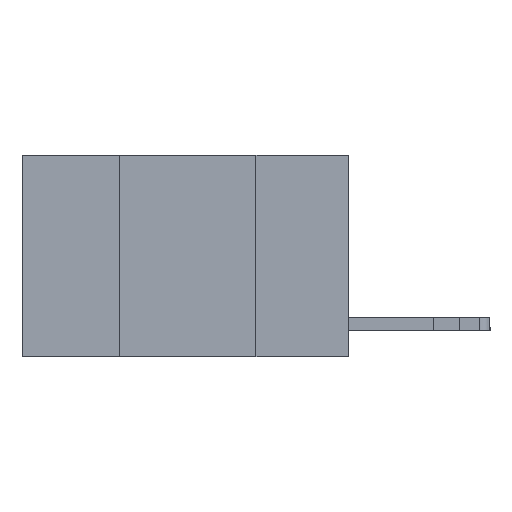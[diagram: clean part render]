
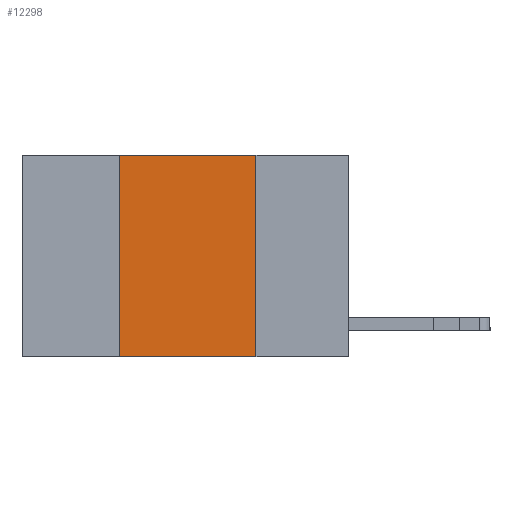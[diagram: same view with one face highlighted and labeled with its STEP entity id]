
A CAD part, left-side view. The second image highlights one B-rep face of the part: STEP entity #12298.
In plain terms, the highlighted planar face has unit normal (-1, 0, 0).
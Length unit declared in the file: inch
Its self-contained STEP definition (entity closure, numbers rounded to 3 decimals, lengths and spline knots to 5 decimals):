
#1018 = ORIENTED_EDGE ( 'NONE', *, *, #19228, .F. ) ;
#1240 = CARTESIAN_POINT ( 'NONE',  ( 0., 0.17, -0.37 ) ) ;
#2890 = VECTOR ( 'NONE', #11458, 39.37008 ) ;
#2961 = ORIENTED_EDGE ( 'NONE', *, *, #23896, .T. ) ;
#3338 = VERTEX_POINT ( 'NONE', #3580 ) ;
#3580 = CARTESIAN_POINT ( 'NONE',  ( 0., 0.42, 0. ) ) ;
#3987 = VERTEX_POINT ( 'NONE', #21225 ) ;
#4457 = FACE_OUTER_BOUND ( 'NONE', #15701, .T. ) ;
#5730 = CARTESIAN_POINT ( 'NONE',  ( 0., 0.6, 0. ) ) ;
#6831 = LINE ( 'NONE', #23111, #14717 ) ;
#6907 = AXIS2_PLACEMENT_3D ( 'NONE', #10648, #14761, #18761 ) ;
#7156 = CARTESIAN_POINT ( 'NONE',  ( 0., 0.6, -0.37 ) ) ;
#9242 = CARTESIAN_POINT ( 'NONE',  ( 0., 0.42, 0. ) ) ;
#10204 = LINE ( 'NONE', #5730, #14156 ) ;
#10648 = CARTESIAN_POINT ( 'NONE',  ( 0., 0.6, 0. ) ) ;
#11253 = CARTESIAN_POINT ( 'NONE',  ( 0., 0.17, 0. ) ) ;
#11458 = DIRECTION ( 'NONE',  ( 0., 0., 1. ) ) ;
#12298 = ADVANCED_FACE ( 'NONE', ( #4457 ), #18889, .F. ) ;
#13047 = LINE ( 'NONE', #9242, #2890 ) ;
#13334 = ORIENTED_EDGE ( 'NONE', *, *, #14646, .F. ) ;
#13776 = DIRECTION ( 'NONE',  ( 0., -1., 0. ) ) ;
#13939 = ORIENTED_EDGE ( 'NONE', *, *, #19636, .F. ) ;
#14156 = VECTOR ( 'NONE', #13776, 39.37008 ) ;
#14543 = VERTEX_POINT ( 'NONE', #11253 ) ;
#14646 = EDGE_CURVE ( 'NONE', #3338, #14543, #10204, .T. ) ;
#14717 = VECTOR ( 'NONE', #14758, 39.37008 ) ;
#14758 = DIRECTION ( 'NONE',  ( 0., 0., -1. ) ) ;
#14761 = DIRECTION ( 'NONE',  ( 1., 0., 0. ) ) ;
#15701 = EDGE_LOOP ( 'NONE', ( #13939, #13334, #1018, #2961 ) ) ;
#16944 = VECTOR ( 'NONE', #25019, 39.37008 ) ;
#18761 = DIRECTION ( 'NONE',  ( 0., 0., -1. ) ) ;
#18889 = PLANE ( 'NONE',  #6907 ) ;
#19228 = EDGE_CURVE ( 'NONE', #3987, #3338, #13047, .T. ) ;
#19636 = EDGE_CURVE ( 'NONE', #14543, #24590, #6831, .T. ) ;
#21225 = CARTESIAN_POINT ( 'NONE',  ( 0., 0.42, -0.37 ) ) ;
#23111 = CARTESIAN_POINT ( 'NONE',  ( 0., 0.17, 0. ) ) ;
#23896 = EDGE_CURVE ( 'NONE', #3987, #24590, #25288, .T. ) ;
#24590 = VERTEX_POINT ( 'NONE', #1240 ) ;
#25019 = DIRECTION ( 'NONE',  ( 0., -1., 0. ) ) ;
#25288 = LINE ( 'NONE', #7156, #16944 ) ;
